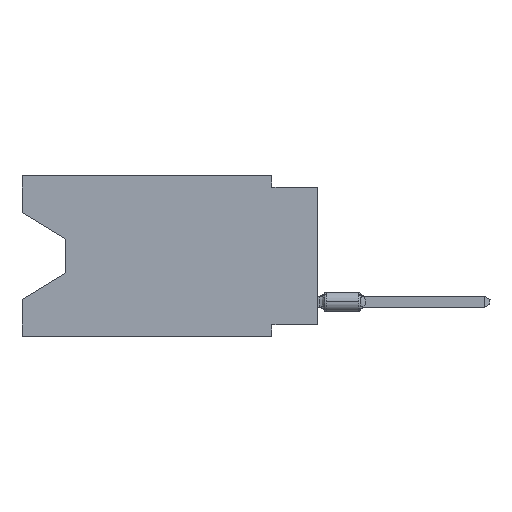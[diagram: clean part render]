
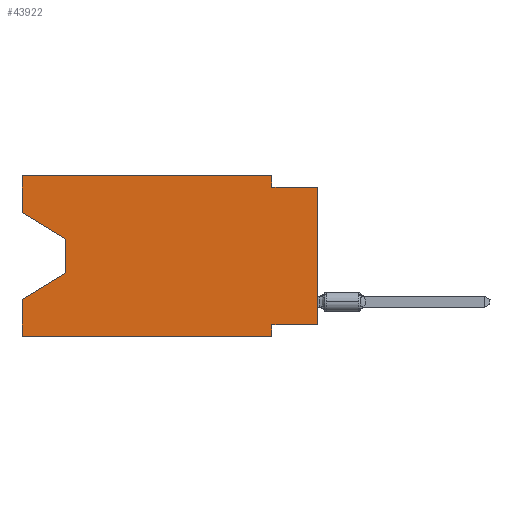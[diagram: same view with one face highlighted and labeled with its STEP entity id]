
A CAD part, left-side view. The second image highlights one B-rep face of the part: STEP entity #43922.
In plain terms, the highlighted planar face has unit normal (-1, 0, 0).
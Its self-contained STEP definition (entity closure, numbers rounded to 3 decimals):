
#331 = ORIENTED_EDGE ( 'NONE', *, *, #67276, .F. ) ;
#504 = VECTOR ( 'NONE', #37430, 1000. ) ;
#1139 = ORIENTED_EDGE ( 'NONE', *, *, #58798, .F. ) ;
#2259 = ORIENTED_EDGE ( 'NONE', *, *, #3750, .F. ) ;
#3243 = DIRECTION ( 'NONE',  ( 0., -0.855, -0.519 ) ) ;
#3750 = EDGE_CURVE ( 'NONE', #4530, #28714, #81215, .T. ) ;
#4006 = CARTESIAN_POINT ( 'NONE',  ( 0., 2.54, -8.255 ) ) ;
#4172 = CARTESIAN_POINT ( 'NONE',  ( 0., 13.97, -5.385 ) ) ;
#4530 = VERTEX_POINT ( 'NONE', #4006 ) ;
#5086 = ORIENTED_EDGE ( 'NONE', *, *, #26235, .T. ) ;
#5155 = VECTOR ( 'NONE', #3243, 1000. ) ;
#5677 = DIRECTION ( 'NONE',  ( 0., 0., -1. ) ) ;
#5698 = CARTESIAN_POINT ( 'NONE',  ( 0., 16.383, -6.852 ) ) ;
#6121 = DIRECTION ( 'NONE',  ( 1., 0., 0. ) ) ;
#6612 = CARTESIAN_POINT ( 'NONE',  ( 0., 16.383, -8.89 ) ) ;
#7111 = CARTESIAN_POINT ( 'NONE',  ( 0., 0., -0.635 ) ) ;
#10656 = CARTESIAN_POINT ( 'NONE',  ( 0., 0., -0.635 ) ) ;
#11061 = CARTESIAN_POINT ( 'NONE',  ( 0., 2.54, 0. ) ) ;
#11763 = VECTOR ( 'NONE', #65613, 1000. ) ;
#12203 = EDGE_CURVE ( 'NONE', #14577, #4530, #34254, .T. ) ;
#12680 = CARTESIAN_POINT ( 'NONE',  ( 0., 16.383, -8.89 ) ) ;
#13237 = CARTESIAN_POINT ( 'NONE',  ( 0., 0., -8.255 ) ) ;
#13591 = ORIENTED_EDGE ( 'NONE', *, *, #17316, .F. ) ;
#13637 = DIRECTION ( 'NONE',  ( 0., 0., -1. ) ) ;
#14577 = VERTEX_POINT ( 'NONE', #13237 ) ;
#15369 = LINE ( 'NONE', #71642, #504 ) ;
#17015 = EDGE_CURVE ( 'NONE', #56206, #28714, #81852, .T. ) ;
#17316 = EDGE_CURVE ( 'NONE', #51105, #52397, #51622, .T. ) ;
#17445 = CARTESIAN_POINT ( 'NONE',  ( 0., 2.54, -0.635 ) ) ;
#18275 = DIRECTION ( 'NONE',  ( 0., 0., -1. ) ) ;
#18635 = DIRECTION ( 'NONE',  ( 0., 0., -1. ) ) ;
#19665 = CARTESIAN_POINT ( 'NONE',  ( 0., 13.97, -3.505 ) ) ;
#19933 = EDGE_CURVE ( 'NONE', #56206, #60701, #43450, .T. ) ;
#20023 = VECTOR ( 'NONE', #29918, 1000. ) ;
#21718 = VECTOR ( 'NONE', #49674, 1000. ) ;
#26180 = ORIENTED_EDGE ( 'NONE', *, *, #76895, .T. ) ;
#26235 = EDGE_CURVE ( 'NONE', #14577, #68836, #53287, .T. ) ;
#27392 = VERTEX_POINT ( 'NONE', #67396 ) ;
#27394 = VECTOR ( 'NONE', #61279, 1000. ) ;
#28714 = VERTEX_POINT ( 'NONE', #41405 ) ;
#29287 = ORIENTED_EDGE ( 'NONE', *, *, #61126, .T. ) ;
#29581 = VECTOR ( 'NONE', #13637, 1000. ) ;
#29918 = DIRECTION ( 'NONE',  ( 0., 0., 1. ) ) ;
#31832 = LINE ( 'NONE', #10656, #11763 ) ;
#33817 = CARTESIAN_POINT ( 'NONE',  ( 0., 0., -8.255 ) ) ;
#34254 = LINE ( 'NONE', #33817, #27394 ) ;
#37430 = DIRECTION ( 'NONE',  ( 0., -1., 0. ) ) ;
#37949 = CARTESIAN_POINT ( 'NONE',  ( 0., 16.383, -2.038 ) ) ;
#38530 = LINE ( 'NONE', #44392, #50941 ) ;
#41121 = CARTESIAN_POINT ( 'NONE',  ( 0., 13.97, -3.505 ) ) ;
#41405 = CARTESIAN_POINT ( 'NONE',  ( 0., 2.54, -8.89 ) ) ;
#43450 = LINE ( 'NONE', #51974, #20023 ) ;
#43922 = ADVANCED_FACE ( 'NONE', ( #87671 ), #60205, .F. ) ;
#44392 = CARTESIAN_POINT ( 'NONE',  ( 0., 13.97, -5.385 ) ) ;
#46093 = DIRECTION ( 'NONE',  ( 0., 0., 1. ) ) ;
#48231 = VERTEX_POINT ( 'NONE', #4172 ) ;
#49674 = DIRECTION ( 'NONE',  ( 0., 0., 1. ) ) ;
#50941 = VECTOR ( 'NONE', #60111, 1000. ) ;
#51105 = VERTEX_POINT ( 'NONE', #85004 ) ;
#51622 = LINE ( 'NONE', #11061, #57294 ) ;
#51974 = CARTESIAN_POINT ( 'NONE',  ( 0., 16.383, 0. ) ) ;
#52397 = VERTEX_POINT ( 'NONE', #17445 ) ;
#53225 = VERTEX_POINT ( 'NONE', #55358 ) ;
#53287 = LINE ( 'NONE', #80311, #59535 ) ;
#54364 = VECTOR ( 'NONE', #88155, 1000. ) ;
#55358 = CARTESIAN_POINT ( 'NONE',  ( 0., 16.383, 0. ) ) ;
#55712 = ORIENTED_EDGE ( 'NONE', *, *, #73120, .F. ) ;
#56206 = VERTEX_POINT ( 'NONE', #12680 ) ;
#57294 = VECTOR ( 'NONE', #18275, 1000. ) ;
#57490 = EDGE_CURVE ( 'NONE', #48231, #60701, #38530, .T. ) ;
#57545 = EDGE_LOOP ( 'NONE', ( #29287, #26180, #78893, #69532, #60679, #2259, #88935, #5086, #331, #13591, #1139, #55712 ) ) ;
#57751 = LINE ( 'NONE', #76690, #21718 ) ;
#58798 = EDGE_CURVE ( 'NONE', #53225, #51105, #15369, .T. ) ;
#59535 = VECTOR ( 'NONE', #46093, 1000. ) ;
#60111 = DIRECTION ( 'NONE',  ( 0., 0.855, -0.519 ) ) ;
#60205 = PLANE ( 'NONE',  #84097 ) ;
#60679 = ORIENTED_EDGE ( 'NONE', *, *, #17015, .T. ) ;
#60701 = VERTEX_POINT ( 'NONE', #5698 ) ;
#61126 = EDGE_CURVE ( 'NONE', #27392, #87108, #87422, .T. ) ;
#61279 = DIRECTION ( 'NONE',  ( 0., 1., 0. ) ) ;
#65613 = DIRECTION ( 'NONE',  ( 0., -1., 0. ) ) ;
#66833 = CARTESIAN_POINT ( 'NONE',  ( 0., 2.54, -8.89 ) ) ;
#67276 = EDGE_CURVE ( 'NONE', #52397, #68836, #31832, .T. ) ;
#67396 = CARTESIAN_POINT ( 'NONE',  ( 0., 16.383, -2.038 ) ) ;
#67404 = CARTESIAN_POINT ( 'NONE',  ( 0., 16.383, 0. ) ) ;
#68836 = VERTEX_POINT ( 'NONE', #7111 ) ;
#69532 = ORIENTED_EDGE ( 'NONE', *, *, #19933, .F. ) ;
#71352 = VECTOR ( 'NONE', #18635, 1000. ) ;
#71642 = CARTESIAN_POINT ( 'NONE',  ( 0., 16.383, 0. ) ) ;
#73120 = EDGE_CURVE ( 'NONE', #27392, #53225, #57751, .T. ) ;
#74440 = LINE ( 'NONE', #41121, #29581 ) ;
#76690 = CARTESIAN_POINT ( 'NONE',  ( 0., 16.383, 0. ) ) ;
#76895 = EDGE_CURVE ( 'NONE', #87108, #48231, #74440, .T. ) ;
#78893 = ORIENTED_EDGE ( 'NONE', *, *, #57490, .T. ) ;
#80311 = CARTESIAN_POINT ( 'NONE',  ( 0., 0., 0. ) ) ;
#81215 = LINE ( 'NONE', #66833, #71352 ) ;
#81852 = LINE ( 'NONE', #6612, #54364 ) ;
#84097 = AXIS2_PLACEMENT_3D ( 'NONE', #67404, #6121, #5677 ) ;
#85004 = CARTESIAN_POINT ( 'NONE',  ( 0., 2.54, 0. ) ) ;
#87108 = VERTEX_POINT ( 'NONE', #19665 ) ;
#87422 = LINE ( 'NONE', #37949, #5155 ) ;
#87671 = FACE_OUTER_BOUND ( 'NONE', #57545, .T. ) ;
#88155 = DIRECTION ( 'NONE',  ( 0., -1., 0. ) ) ;
#88935 = ORIENTED_EDGE ( 'NONE', *, *, #12203, .F. ) ;
